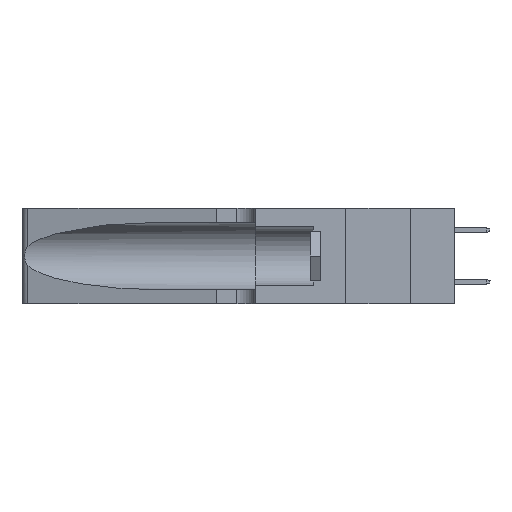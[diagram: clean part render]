
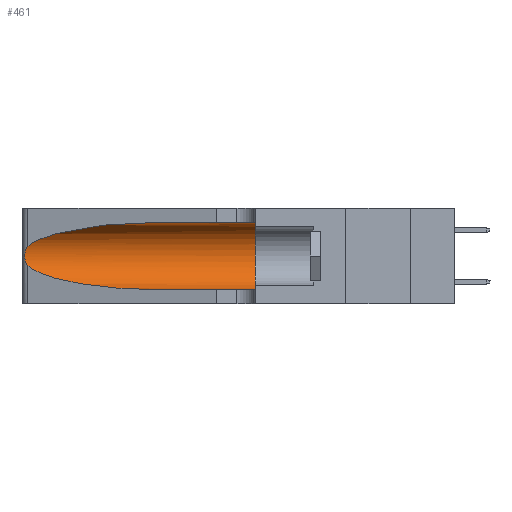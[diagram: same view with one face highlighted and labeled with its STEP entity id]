
A CAD part, left-side view. The second image highlights one B-rep face of the part: STEP entity #461.
In plain terms, the highlighted cylindrical face has radius 3.308 mm (diameter 6.617 mm), a partial arc.
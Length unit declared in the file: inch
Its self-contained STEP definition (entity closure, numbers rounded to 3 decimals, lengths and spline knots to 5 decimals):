
#99 = FACE_OUTER_BOUND ( 'NONE', #23138, .T. ) ;
#262 = CARTESIAN_POINT ( 'NONE',  ( 0.1305, 1.61858, 0.05475 ) ) ;
#461 = ADVANCED_FACE ( 'NONE', ( #99 ), #6819, .F. ) ;
#1504 = VECTOR ( 'NONE', #20380, 39.37008 ) ;
#2051 = CARTESIAN_POINT ( 'NONE',  ( 0.2373, 1.15595, 0.28018 ) ) ;
#2347 = ORIENTED_EDGE ( 'NONE', *, *, #5561, .T. ) ;
#2707 = CARTESIAN_POINT ( 'NONE',  ( 0.26075, 1.23896, 0.178 ) ) ;
#2949 = VECTOR ( 'NONE', #26503, 39.37008 ) ;
#2959 = EDGE_CURVE ( 'NONE', #26448, #19888, #25466, .T. ) ;
#3254 = CARTESIAN_POINT ( 'NONE',  ( 0.25787, 1.23484, 0.2124 ) ) ;
#3424 = ORIENTED_EDGE ( 'NONE', *, *, #27412, .T. ) ;
#3920 = VERTEX_POINT ( 'NONE', #15429 ) ;
#4177 = CARTESIAN_POINT ( 'NONE',  ( 0.1305, 0.72297, 0.31525 ) ) ;
#4204 = DIRECTION ( 'NONE',  ( 0., 0., 1. ) ) ;
#4745 = ORIENTED_EDGE ( 'NONE', *, *, #2959, .F. ) ;
#4940 = VERTEX_POINT ( 'NONE', #18000 ) ;
#5304 = ORIENTED_EDGE ( 'NONE', *, *, #14561, .F. ) ;
#5366 = CARTESIAN_POINT ( 'NONE',  ( 0.2373, 1.15595, 0.08982 ) ) ;
#5394 = AXIS2_PLACEMENT_3D ( 'NONE', #19919, #21916, #12770 ) ;
#5453 =( BOUNDED_CURVE ( )  B_SPLINE_CURVE ( 3, ( #4177, #12856, #2051, #10706 ),
 .UNSPECIFIED., .F., .T. ) 
 B_SPLINE_CURVE_WITH_KNOTS ( ( 4, 4 ),
 ( 1.5708, 2.84003 ),
 .UNSPECIFIED. ) 
 CURVE ( )  GEOMETRIC_REPRESENTATION_ITEM ( )  RATIONAL_B_SPLINE_CURVE ( ( 1., 0.87, 0.87, 1. ) ) 
 REPRESENTATION_ITEM ( '' )  );
#5561 = EDGE_CURVE ( 'NONE', #19582, #10222, #22030, .T. ) ;
#6819 = CYLINDRICAL_SURFACE ( 'NONE', #5394, 0.13025 ) ;
#7520 = CARTESIAN_POINT ( 'NONE',  ( 0.25487, 1.22718, 0.14631 ) ) ;
#7532 = CARTESIAN_POINT ( 'NONE',  ( 0.25487, 1.22718, 0.22369 ) ) ;
#7668 = CARTESIAN_POINT ( 'NONE',  ( 0.25789, 1.23486, 0.15765 ) ) ;
#9746 = CARTESIAN_POINT ( 'NONE',  ( 0.25487, 1.22718, 0.14631 ) ) ;
#10151 = EDGE_CURVE ( 'NONE', #4940, #19582, #20028, .T. ) ;
#10222 = VERTEX_POINT ( 'NONE', #27626 ) ;
#10706 = CARTESIAN_POINT ( 'NONE',  ( 0.25487, 1.22718, 0.22369 ) ) ;
#10869 = AXIS2_PLACEMENT_3D ( 'NONE', #21313, #23748, #4204 ) ;
#11374 = CARTESIAN_POINT ( 'NONE',  ( 0.25555, 1.22993, 0.14849 ) ) ;
#11633 = CARTESIAN_POINT ( 'NONE',  ( 0.1305, 0.72297, 0.05475 ) ) ;
#11930 = CARTESIAN_POINT ( 'NONE',  ( 0.25854, 1.2359, 0.20912 ) ) ;
#12770 = DIRECTION ( 'NONE',  ( 0., 0., -1. ) ) ;
#12856 = CARTESIAN_POINT ( 'NONE',  ( 0.18966, 0.96281, 0.31525 ) ) ;
#13165 = ORIENTED_EDGE ( 'NONE', *, *, #10151, .T. ) ;
#13475 = CARTESIAN_POINT ( 'NONE',  ( 0.25639, 1.23186, 0.15144 ) ) ;
#13801 = CARTESIAN_POINT ( 'NONE',  ( 0.1305, 1.61858, 0.31525 ) ) ;
#14030 = CARTESIAN_POINT ( 'NONE',  ( 0.18966, 0.96281, 0.05475 ) ) ;
#14049 = CARTESIAN_POINT ( 'NONE',  ( 0.25555, 1.22994, 0.2215 ) ) ;
#14561 = EDGE_CURVE ( 'NONE', #3920, #26448, #15937, .T. ) ;
#15429 = CARTESIAN_POINT ( 'NONE',  ( 0.1305, 0.72297, 0.31525 ) ) ;
#15937 = LINE ( 'NONE', #13801, #1504 ) ;
#15964 = EDGE_CURVE ( 'NONE', #10222, #19888, #19658, .T. ) ;
#16148 = ORIENTED_EDGE ( 'NONE', *, *, #15964, .T. ) ;
#18000 = CARTESIAN_POINT ( 'NONE',  ( 0.25487, 1.22718, 0.22369 ) ) ;
#18466 = CARTESIAN_POINT ( 'NONE',  ( 0.26017, 1.23833, 0.17102 ) ) ;
#18966 = CARTESIAN_POINT ( 'NONE',  ( 0.1305, 0.35, 0.31525 ) ) ;
#19582 = VERTEX_POINT ( 'NONE', #9746 ) ;
#19658 = LINE ( 'NONE', #262, #2949 ) ;
#19888 = VERTEX_POINT ( 'NONE', #20410 ) ;
#19919 = CARTESIAN_POINT ( 'NONE',  ( 0.1305, 1.61858, 0.185 ) ) ;
#20028 = B_SPLINE_CURVE_WITH_KNOTS ( 'NONE', 3,
 ( #7532, #14049, #22776, #3254, #11930, #25053, #20633, #2707, #18466, #27195, #7668, #13475, #11374, #20083 ),
 .UNSPECIFIED., .F., .F.,
 ( 4, 2, 2, 2, 2, 2, 4 ),
 ( 0., 0.00027, 0.00053, 0.00107, 0.0016, 0.00187, 0.00214 ),
 .UNSPECIFIED. ) ;
#20083 = CARTESIAN_POINT ( 'NONE',  ( 0.25487, 1.22718, 0.14631 ) ) ;
#20380 = DIRECTION ( 'NONE',  ( 0., -1., 0. ) ) ;
#20410 = CARTESIAN_POINT ( 'NONE',  ( 0.1305, 0.35, 0.05475 ) ) ;
#20633 = CARTESIAN_POINT ( 'NONE',  ( 0.26075, 1.23896, 0.19203 ) ) ;
#21313 = CARTESIAN_POINT ( 'NONE',  ( 0.1305, 0.35, 0.185 ) ) ;
#21916 = DIRECTION ( 'NONE',  ( 0., -1., 0. ) ) ;
#22030 =( BOUNDED_CURVE ( )  B_SPLINE_CURVE ( 3, ( #7520, #5366, #14030, #11633 ),
 .UNSPECIFIED., .F., .T. ) 
 B_SPLINE_CURVE_WITH_KNOTS ( ( 4, 4 ),
 ( 3.44316, 4.71239 ),
 .UNSPECIFIED. ) 
 CURVE ( )  GEOMETRIC_REPRESENTATION_ITEM ( )  RATIONAL_B_SPLINE_CURVE ( ( 1., 0.87, 0.87, 1. ) ) 
 REPRESENTATION_ITEM ( '' )  );
#22776 = CARTESIAN_POINT ( 'NONE',  ( 0.25639, 1.23184, 0.21858 ) ) ;
#23138 = EDGE_LOOP ( 'NONE', ( #3424, #13165, #2347, #16148, #4745, #5304 ) ) ;
#23748 = DIRECTION ( 'NONE',  ( 0., 1., 0. ) ) ;
#25053 = CARTESIAN_POINT ( 'NONE',  ( 0.26018, 1.23835, 0.19895 ) ) ;
#25466 = CIRCLE ( 'NONE', #10869, 0.13025 ) ;
#26448 = VERTEX_POINT ( 'NONE', #18966 ) ;
#26503 = DIRECTION ( 'NONE',  ( 0., -1., 0. ) ) ;
#27195 = CARTESIAN_POINT ( 'NONE',  ( 0.25856, 1.23593, 0.16098 ) ) ;
#27412 = EDGE_CURVE ( 'NONE', #3920, #4940, #5453, .T. ) ;
#27626 = CARTESIAN_POINT ( 'NONE',  ( 0.1305, 0.72297, 0.05475 ) ) ;
